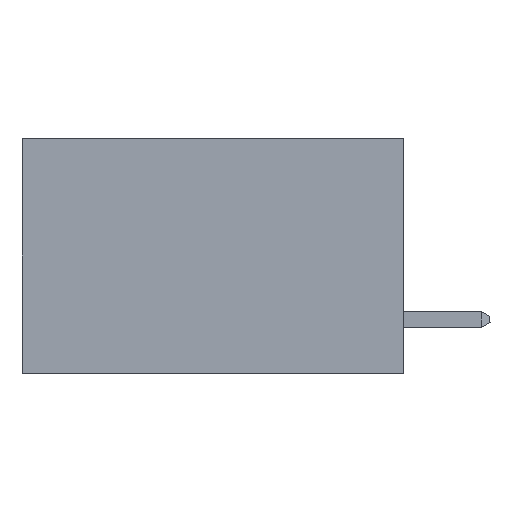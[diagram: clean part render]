
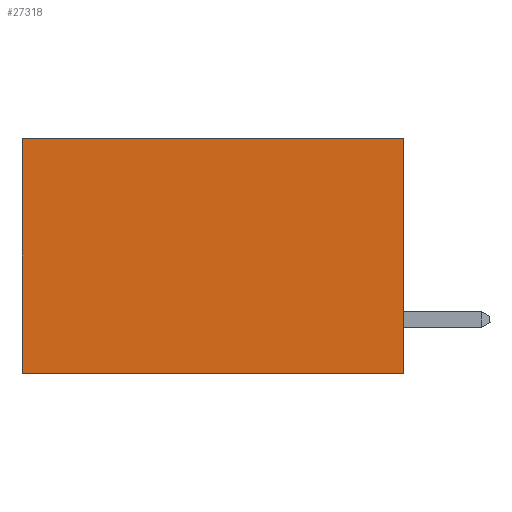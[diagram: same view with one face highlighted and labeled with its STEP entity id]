
A CAD part, left-side view. The second image highlights one B-rep face of the part: STEP entity #27318.
In plain terms, the highlighted planar face has unit normal (-1, 0, 0).
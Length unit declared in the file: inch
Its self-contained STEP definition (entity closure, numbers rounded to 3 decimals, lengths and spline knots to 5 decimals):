
#1844 = VECTOR ( 'NONE', #22032, 39.37008 ) ;
#2395 = CARTESIAN_POINT ( 'NONE',  ( 0.2875, 0., -0.37 ) ) ;
#2742 = LINE ( 'NONE', #10667, #3123 ) ;
#3123 = VECTOR ( 'NONE', #17124, 39.37008 ) ;
#4527 = CARTESIAN_POINT ( 'NONE',  ( 0.2875, 0.6, -0.37 ) ) ;
#6573 = LINE ( 'NONE', #23932, #15772 ) ;
#6744 = CARTESIAN_POINT ( 'NONE',  ( 0.2875, 0., 0. ) ) ;
#9704 = CARTESIAN_POINT ( 'NONE',  ( 0.2875, 0., 0. ) ) ;
#9905 = DIRECTION ( 'NONE',  ( 0., 0., -1. ) ) ;
#10667 = CARTESIAN_POINT ( 'NONE',  ( 0.2875, 0.6, 0. ) ) ;
#12452 = EDGE_CURVE ( 'NONE', #17646, #17702, #2742, .T. ) ;
#12988 = VERTEX_POINT ( 'NONE', #15658 ) ;
#13903 = LINE ( 'NONE', #6744, #14239 ) ;
#14239 = VECTOR ( 'NONE', #22242, 39.37008 ) ;
#15658 = CARTESIAN_POINT ( 'NONE',  ( 0.2875, 0., 0. ) ) ;
#15772 = VECTOR ( 'NONE', #18165, 39.37008 ) ;
#16344 = CARTESIAN_POINT ( 'NONE',  ( 0.2875, 0.6, 0. ) ) ;
#17124 = DIRECTION ( 'NONE',  ( 0., 0., -1. ) ) ;
#17646 = VERTEX_POINT ( 'NONE', #16344 ) ;
#17702 = VERTEX_POINT ( 'NONE', #4527 ) ;
#17769 = ORIENTED_EDGE ( 'NONE', *, *, #23395, .T. ) ;
#18015 = VERTEX_POINT ( 'NONE', #2395 ) ;
#18077 = ORIENTED_EDGE ( 'NONE', *, *, #26209, .F. ) ;
#18165 = DIRECTION ( 'NONE',  ( 0., 0., -1. ) ) ;
#19894 = AXIS2_PLACEMENT_3D ( 'NONE', #9704, #27234, #9905 ) ;
#20369 = PLANE ( 'NONE',  #19894 ) ;
#20411 = EDGE_CURVE ( 'NONE', #12988, #18015, #6573, .T. ) ;
#22032 = DIRECTION ( 'NONE',  ( 0., 1., 0. ) ) ;
#22242 = DIRECTION ( 'NONE',  ( 0., 1., 0. ) ) ;
#23327 = ORIENTED_EDGE ( 'NONE', *, *, #20411, .F. ) ;
#23395 = EDGE_CURVE ( 'NONE', #12988, #17646, #13903, .T. ) ;
#23932 = CARTESIAN_POINT ( 'NONE',  ( 0.2875, 0., 0. ) ) ;
#25731 = LINE ( 'NONE', #26325, #1844 ) ;
#25932 = EDGE_LOOP ( 'NONE', ( #26969, #18077, #23327, #17769 ) ) ;
#26209 = EDGE_CURVE ( 'NONE', #18015, #17702, #25731, .T. ) ;
#26325 = CARTESIAN_POINT ( 'NONE',  ( 0.2875, 0., -0.37 ) ) ;
#26969 = ORIENTED_EDGE ( 'NONE', *, *, #12452, .T. ) ;
#27234 = DIRECTION ( 'NONE',  ( 1., 0., 0. ) ) ;
#27318 = ADVANCED_FACE ( 'NONE', ( #28059 ), #20369, .F. ) ;
#28059 = FACE_OUTER_BOUND ( 'NONE', #25932, .T. ) ;
